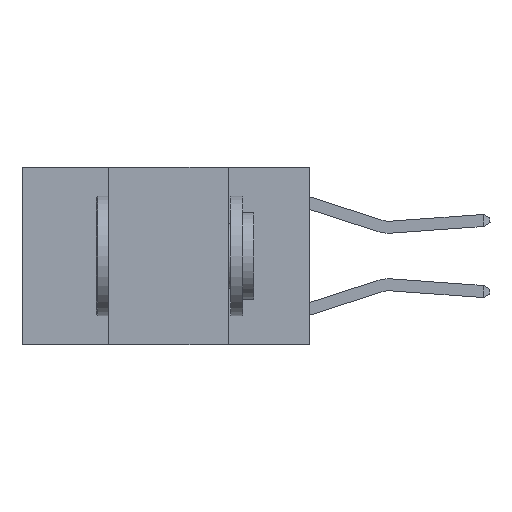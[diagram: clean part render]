
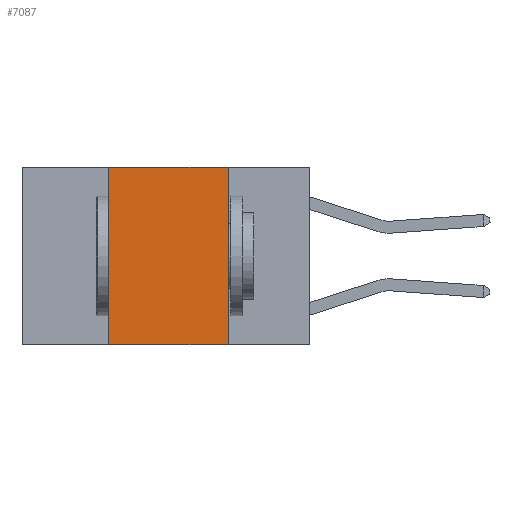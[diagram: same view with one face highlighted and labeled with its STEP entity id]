
A CAD part, left-side view. The second image highlights one B-rep face of the part: STEP entity #7087.
In plain terms, the highlighted planar face has unit normal (-1, 0, 0).
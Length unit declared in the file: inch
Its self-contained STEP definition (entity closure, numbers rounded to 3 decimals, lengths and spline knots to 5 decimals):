
#472 = ORIENTED_EDGE ( 'NONE', *, *, #4279, .F. ) ;
#955 = EDGE_LOOP ( 'NONE', ( #8103, #472, #8977, #7939 ) ) ;
#1035 = PLANE ( 'NONE',  #9316 ) ;
#1656 = EDGE_CURVE ( 'NONE', #5764, #4438, #5501, .T. ) ;
#1715 = EDGE_CURVE ( 'NONE', #5764, #5589, #2106, .T. ) ;
#1811 = DIRECTION ( 'NONE',  ( 0., 0., -1. ) ) ;
#2038 = LINE ( 'NONE', #4545, #6452 ) ;
#2106 = LINE ( 'NONE', #6845, #6282 ) ;
#2864 = EDGE_CURVE ( 'NONE', #9886, #5589, #6947, .T. ) ;
#4279 = EDGE_CURVE ( 'NONE', #4438, #9886, #2038, .T. ) ;
#4438 = VERTEX_POINT ( 'NONE', #7958 ) ;
#4545 = CARTESIAN_POINT ( 'NONE',  ( 0., 0.6, 0. ) ) ;
#5354 = DIRECTION ( 'NONE',  ( 0., 0., -1. ) ) ;
#5444 = CARTESIAN_POINT ( 'NONE',  ( 0., 0.17, -0.37 ) ) ;
#5501 = LINE ( 'NONE', #6471, #9212 ) ;
#5589 = VERTEX_POINT ( 'NONE', #5444 ) ;
#5655 = CARTESIAN_POINT ( 'NONE',  ( 0., 0.17, 0. ) ) ;
#5764 = VERTEX_POINT ( 'NONE', #7107 ) ;
#6282 = VECTOR ( 'NONE', #8293, 39.37008 ) ;
#6452 = VECTOR ( 'NONE', #9834, 39.37008 ) ;
#6471 = CARTESIAN_POINT ( 'NONE',  ( 0., 0.42, 0. ) ) ;
#6607 = DIRECTION ( 'NONE',  ( 0., 0., 1. ) ) ;
#6694 = FACE_OUTER_BOUND ( 'NONE', #955, .T. ) ;
#6739 = DIRECTION ( 'NONE',  ( 1., 0., 0. ) ) ;
#6845 = CARTESIAN_POINT ( 'NONE',  ( 0., 0.6, -0.37 ) ) ;
#6947 = LINE ( 'NONE', #5655, #8706 ) ;
#7087 = ADVANCED_FACE ( 'NONE', ( #6694 ), #1035, .F. ) ;
#7107 = CARTESIAN_POINT ( 'NONE',  ( 0., 0.42, -0.37 ) ) ;
#7466 = CARTESIAN_POINT ( 'NONE',  ( 0., 0.6, 0. ) ) ;
#7939 = ORIENTED_EDGE ( 'NONE', *, *, #1715, .T. ) ;
#7958 = CARTESIAN_POINT ( 'NONE',  ( 0., 0.42, 0. ) ) ;
#8103 = ORIENTED_EDGE ( 'NONE', *, *, #2864, .F. ) ;
#8293 = DIRECTION ( 'NONE',  ( 0., -1., 0. ) ) ;
#8706 = VECTOR ( 'NONE', #5354, 39.37008 ) ;
#8977 = ORIENTED_EDGE ( 'NONE', *, *, #1656, .F. ) ;
#9212 = VECTOR ( 'NONE', #6607, 39.37008 ) ;
#9316 = AXIS2_PLACEMENT_3D ( 'NONE', #7466, #6739, #1811 ) ;
#9368 = CARTESIAN_POINT ( 'NONE',  ( 0., 0.17, 0. ) ) ;
#9834 = DIRECTION ( 'NONE',  ( 0., -1., 0. ) ) ;
#9886 = VERTEX_POINT ( 'NONE', #9368 ) ;
